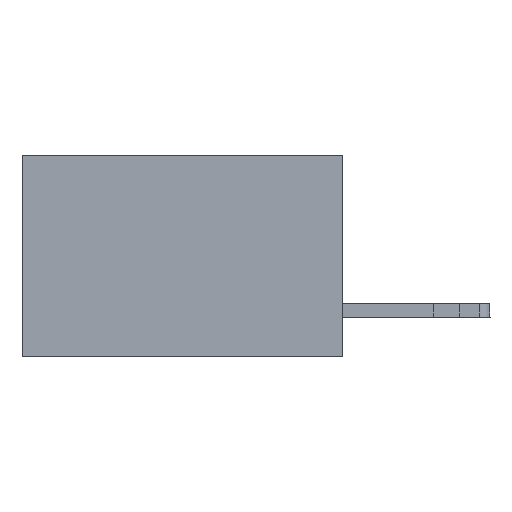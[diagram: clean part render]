
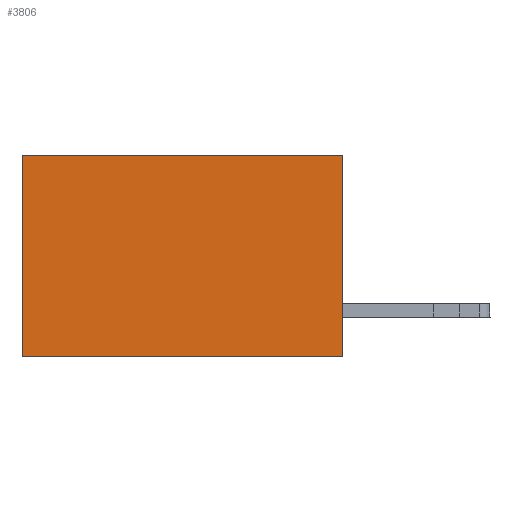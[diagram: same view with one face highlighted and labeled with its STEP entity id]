
A CAD part, left-side view. The second image highlights one B-rep face of the part: STEP entity #3806.
In plain terms, the highlighted planar face has unit normal (-1, 0, 0).
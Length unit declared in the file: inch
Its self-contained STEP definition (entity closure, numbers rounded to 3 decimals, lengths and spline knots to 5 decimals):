
#89 = CARTESIAN_POINT ( 'NONE',  ( 0.277, 0., -0.37 ) ) ;
#704 = CARTESIAN_POINT ( 'NONE',  ( 0.277, 0., -0.37 ) ) ;
#1648 = VERTEX_POINT ( 'NONE', #89 ) ;
#1847 = VECTOR ( 'NONE', #16907, 39.37008 ) ;
#2139 = CARTESIAN_POINT ( 'NONE',  ( 0.277, 0.59, 0. ) ) ;
#2987 = LINE ( 'NONE', #9523, #5415 ) ;
#3806 = ADVANCED_FACE ( 'NONE', ( #12042 ), #17277, .F. ) ;
#4478 = EDGE_CURVE ( 'NONE', #12055, #15260, #11998, .T. ) ;
#5318 = LINE ( 'NONE', #11947, #12266 ) ;
#5415 = VECTOR ( 'NONE', #13949, 39.37008 ) ;
#5496 = AXIS2_PLACEMENT_3D ( 'NONE', #12219, #14791, #10709 ) ;
#6067 = VECTOR ( 'NONE', #16156, 39.37008 ) ;
#6368 = LINE ( 'NONE', #704, #1847 ) ;
#8017 = CARTESIAN_POINT ( 'NONE',  ( 0.277, 0., 0. ) ) ;
#8144 = DIRECTION ( 'NONE',  ( 0., 0., -1. ) ) ;
#8152 = EDGE_LOOP ( 'NONE', ( #10128, #15722, #8426, #15985 ) ) ;
#8426 = ORIENTED_EDGE ( 'NONE', *, *, #11901, .F. ) ;
#9523 = CARTESIAN_POINT ( 'NONE',  ( 0.277, 0., -0.37 ) ) ;
#10128 = ORIENTED_EDGE ( 'NONE', *, *, #16717, .T. ) ;
#10709 = DIRECTION ( 'NONE',  ( 0., 0., -1. ) ) ;
#11901 = EDGE_CURVE ( 'NONE', #12055, #1648, #2987, .T. ) ;
#11947 = CARTESIAN_POINT ( 'NONE',  ( 0.277, 0.59, -0.37 ) ) ;
#11998 = LINE ( 'NONE', #8017, #6067 ) ;
#12042 = FACE_OUTER_BOUND ( 'NONE', #8152, .T. ) ;
#12055 = VERTEX_POINT ( 'NONE', #12975 ) ;
#12219 = CARTESIAN_POINT ( 'NONE',  ( 0.277, 0., -0.37 ) ) ;
#12266 = VECTOR ( 'NONE', #8144, 39.37008 ) ;
#12975 = CARTESIAN_POINT ( 'NONE',  ( 0.277, 0., 0. ) ) ;
#13813 = VERTEX_POINT ( 'NONE', #15283 ) ;
#13949 = DIRECTION ( 'NONE',  ( 0., 0., -1. ) ) ;
#14791 = DIRECTION ( 'NONE',  ( 1., 0., 0. ) ) ;
#15260 = VERTEX_POINT ( 'NONE', #2139 ) ;
#15283 = CARTESIAN_POINT ( 'NONE',  ( 0.277, 0.59, -0.37 ) ) ;
#15722 = ORIENTED_EDGE ( 'NONE', *, *, #17056, .F. ) ;
#15985 = ORIENTED_EDGE ( 'NONE', *, *, #4478, .T. ) ;
#16156 = DIRECTION ( 'NONE',  ( 0., 1., 0. ) ) ;
#16717 = EDGE_CURVE ( 'NONE', #15260, #13813, #5318, .T. ) ;
#16907 = DIRECTION ( 'NONE',  ( 0., 1., 0. ) ) ;
#17056 = EDGE_CURVE ( 'NONE', #1648, #13813, #6368, .T. ) ;
#17277 = PLANE ( 'NONE',  #5496 ) ;
